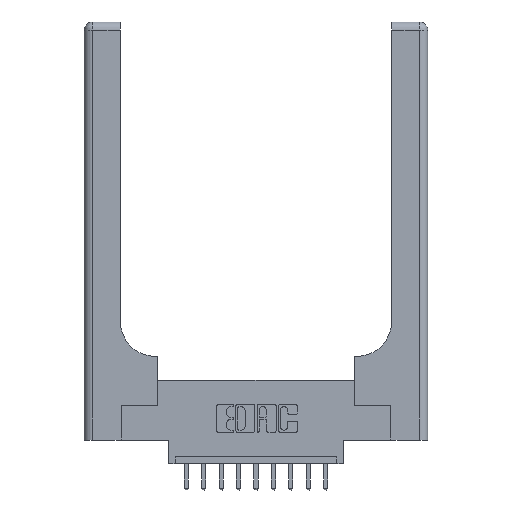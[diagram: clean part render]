
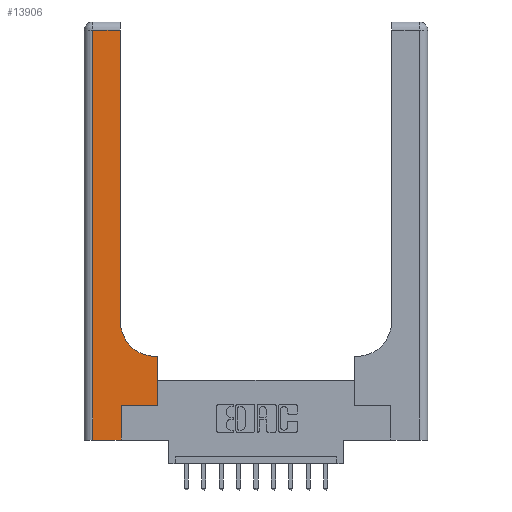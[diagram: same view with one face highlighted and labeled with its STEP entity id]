
A CAD part, top view. The second image highlights one B-rep face of the part: STEP entity #13906.
In plain terms, the highlighted planar face has unit normal (0, 0, 1).
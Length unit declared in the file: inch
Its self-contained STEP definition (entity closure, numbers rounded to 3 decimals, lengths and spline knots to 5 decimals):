
#676 = DIRECTION ( 'NONE',  ( 1., 0., 0. ) ) ;
#1012 = EDGE_CURVE ( 'NONE', #5408, #9602, #3249, .T. ) ;
#1483 = CARTESIAN_POINT ( 'NONE',  ( 0.26, 3., 0.37 ) ) ;
#1623 = LINE ( 'NONE', #14993, #15176 ) ;
#1718 = VERTEX_POINT ( 'NONE', #3840 ) ;
#1794 = AXIS2_PLACEMENT_3D ( 'NONE', #9334, #3446, #8146 ) ;
#1863 = DIRECTION ( 'NONE',  ( 0., 1., 0. ) ) ;
#2030 = LINE ( 'NONE', #6917, #14494 ) ;
#2334 = ORIENTED_EDGE ( 'NONE', *, *, #9064, .T. ) ;
#2750 = VERTEX_POINT ( 'NONE', #8456 ) ;
#2884 = ORIENTED_EDGE ( 'NONE', *, *, #15511, .T. ) ;
#3249 = LINE ( 'NONE', #3326, #11176 ) ;
#3326 = CARTESIAN_POINT ( 'NONE',  ( 0., 2.94, 0.37 ) ) ;
#3446 = DIRECTION ( 'NONE',  ( 0., 0., -1. ) ) ;
#3633 = CARTESIAN_POINT ( 'NONE',  ( 0.265, 0., 0.37 ) ) ;
#3840 = CARTESIAN_POINT ( 'NONE',  ( 0.265, 0., 0.37 ) ) ;
#3882 = ORIENTED_EDGE ( 'NONE', *, *, #1012, .T. ) ;
#4061 = ORIENTED_EDGE ( 'NONE', *, *, #6616, .T. ) ;
#4330 = VECTOR ( 'NONE', #6363, 39.37008 ) ;
#4385 = EDGE_LOOP ( 'NONE', ( #2334, #3882, #2884, #15299, #12200, #11064, #4061, #10238, #8839 ) ) ;
#4434 = AXIS2_PLACEMENT_3D ( 'NONE', #9200, #5639, #8087 ) ;
#4795 = DIRECTION ( 'NONE',  ( 1., 0., 0. ) ) ;
#4809 = CARTESIAN_POINT ( 'NONE',  ( 0.528, 0.25, 0.37 ) ) ;
#5408 = VERTEX_POINT ( 'NONE', #14054 ) ;
#5479 = EDGE_CURVE ( 'NONE', #2750, #15726, #11777, .T. ) ;
#5617 = EDGE_CURVE ( 'NONE', #7703, #1718, #15695, .T. ) ;
#5639 = DIRECTION ( 'NONE',  ( 0., 0., -1. ) ) ;
#5715 = FACE_OUTER_BOUND ( 'NONE', #4385, .T. ) ;
#6363 = DIRECTION ( 'NONE',  ( 0., 1., 0. ) ) ;
#6616 = EDGE_CURVE ( 'NONE', #15726, #7915, #1623, .T. ) ;
#6917 = CARTESIAN_POINT ( 'NONE',  ( 0.06, 3., 0.37 ) ) ;
#7461 = CARTESIAN_POINT ( 'NONE',  ( 0.26, 0.6, 0.37 ) ) ;
#7482 = CARTESIAN_POINT ( 'NONE',  ( 0.06, 0., 0.37 ) ) ;
#7681 = VERTEX_POINT ( 'NONE', #10956 ) ;
#7703 = VERTEX_POINT ( 'NONE', #7482 ) ;
#7915 = VERTEX_POINT ( 'NONE', #14058 ) ;
#7978 = EDGE_CURVE ( 'NONE', #11266, #7681, #11040, .T. ) ;
#8087 = DIRECTION ( 'NONE',  ( -1., 0., 0. ) ) ;
#8146 = DIRECTION ( 'NONE',  ( 1., 0., 0. ) ) ;
#8197 = EDGE_CURVE ( 'NONE', #7915, #11266, #13550, .T. ) ;
#8251 = DIRECTION ( 'NONE',  ( -1., 0., 0. ) ) ;
#8456 = CARTESIAN_POINT ( 'NONE',  ( 0.265, 0.25, 0.37 ) ) ;
#8839 = ORIENTED_EDGE ( 'NONE', *, *, #7978, .T. ) ;
#9021 = VECTOR ( 'NONE', #4795, 39.37008 ) ;
#9064 = EDGE_CURVE ( 'NONE', #7681, #5408, #12528, .T. ) ;
#9200 = CARTESIAN_POINT ( 'NONE',  ( 0., 3., 0.37 ) ) ;
#9334 = CARTESIAN_POINT ( 'NONE',  ( 0.51, 0.85, 0.37 ) ) ;
#9602 = VERTEX_POINT ( 'NONE', #12611 ) ;
#9756 = DIRECTION ( 'NONE',  ( 0., 1., 0. ) ) ;
#9911 = CARTESIAN_POINT ( 'NONE',  ( 0.51, 0.6, 0.37 ) ) ;
#10238 = ORIENTED_EDGE ( 'NONE', *, *, #8197, .T. ) ;
#10634 = DIRECTION ( 'NONE',  ( 0., -1., 0. ) ) ;
#10956 = CARTESIAN_POINT ( 'NONE',  ( 0.26, 0.85, 0.37 ) ) ;
#10971 = LINE ( 'NONE', #3633, #14736 ) ;
#11040 = CIRCLE ( 'NONE', #1794, 0.25 ) ;
#11064 = ORIENTED_EDGE ( 'NONE', *, *, #5479, .T. ) ;
#11096 = CARTESIAN_POINT ( 'NONE',  ( 0., 0., 0.37 ) ) ;
#11176 = VECTOR ( 'NONE', #8251, 39.37008 ) ;
#11261 = DIRECTION ( 'NONE',  ( -1., 0., 0. ) ) ;
#11266 = VERTEX_POINT ( 'NONE', #9911 ) ;
#11536 = VECTOR ( 'NONE', #676, 39.37008 ) ;
#11777 = LINE ( 'NONE', #14424, #11536 ) ;
#12200 = ORIENTED_EDGE ( 'NONE', *, *, #15188, .T. ) ;
#12528 = LINE ( 'NONE', #1483, #4330 ) ;
#12611 = CARTESIAN_POINT ( 'NONE',  ( 0.06, 2.94, 0.37 ) ) ;
#12836 = VECTOR ( 'NONE', #11261, 39.37008 ) ;
#13550 = LINE ( 'NONE', #7461, #12836 ) ;
#13906 = ADVANCED_FACE ( 'NONE', ( #5715 ), #15575, .F. ) ;
#14054 = CARTESIAN_POINT ( 'NONE',  ( 0.26, 2.94, 0.37 ) ) ;
#14058 = CARTESIAN_POINT ( 'NONE',  ( 0.528, 0.6, 0.37 ) ) ;
#14424 = CARTESIAN_POINT ( 'NONE',  ( 0.265, 0.25, 0.37 ) ) ;
#14494 = VECTOR ( 'NONE', #10634, 39.37008 ) ;
#14736 = VECTOR ( 'NONE', #9756, 39.37008 ) ;
#14993 = CARTESIAN_POINT ( 'NONE',  ( 0.528, 0.25, 0.37 ) ) ;
#15176 = VECTOR ( 'NONE', #1863, 39.37008 ) ;
#15188 = EDGE_CURVE ( 'NONE', #1718, #2750, #10971, .T. ) ;
#15299 = ORIENTED_EDGE ( 'NONE', *, *, #5617, .T. ) ;
#15511 = EDGE_CURVE ( 'NONE', #9602, #7703, #2030, .T. ) ;
#15575 = PLANE ( 'NONE',  #4434 ) ;
#15695 = LINE ( 'NONE', #11096, #9021 ) ;
#15726 = VERTEX_POINT ( 'NONE', #4809 ) ;
